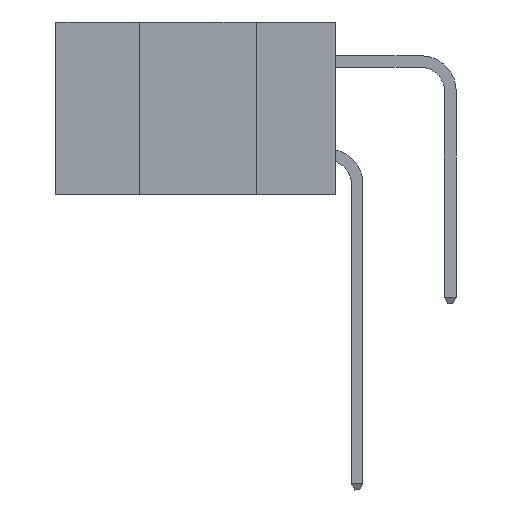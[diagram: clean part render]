
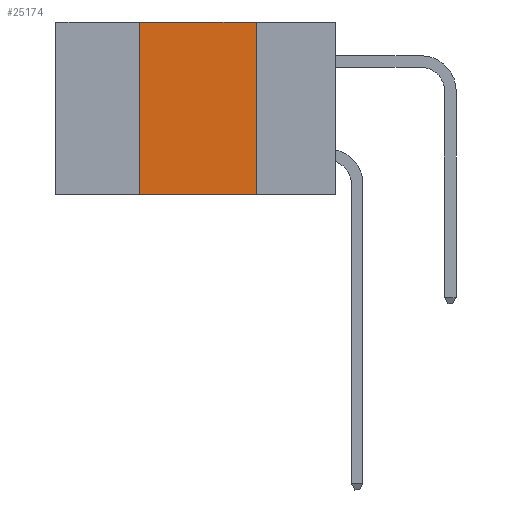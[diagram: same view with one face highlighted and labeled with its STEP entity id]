
A CAD part, left-side view. The second image highlights one B-rep face of the part: STEP entity #25174.
In plain terms, the highlighted planar face has unit normal (-1, 0, 0).
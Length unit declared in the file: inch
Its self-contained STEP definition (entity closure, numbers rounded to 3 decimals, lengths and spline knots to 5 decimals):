
#180 = CARTESIAN_POINT ( 'NONE',  ( 0., 0.42, -0.37 ) ) ;
#3259 = FACE_OUTER_BOUND ( 'NONE', #9190, .T. ) ;
#3650 = AXIS2_PLACEMENT_3D ( 'NONE', #17497, #11956, #22484 ) ;
#5127 = DIRECTION ( 'NONE',  ( 0., 0., -1. ) ) ;
#6590 = CARTESIAN_POINT ( 'NONE',  ( 0., 0.6, 0. ) ) ;
#7867 = LINE ( 'NONE', #29568, #27215 ) ;
#8595 = VERTEX_POINT ( 'NONE', #17747 ) ;
#9190 = EDGE_LOOP ( 'NONE', ( #14017, #14100, #24535, #16120 ) ) ;
#11164 = VECTOR ( 'NONE', #32079, 39.37008 ) ;
#11956 = DIRECTION ( 'NONE',  ( 1., 0., 0. ) ) ;
#12227 = EDGE_CURVE ( 'NONE', #27423, #13908, #7867, .T. ) ;
#12720 = CARTESIAN_POINT ( 'NONE',  ( 0., 0.17, 0. ) ) ;
#13908 = VERTEX_POINT ( 'NONE', #24430 ) ;
#14017 = ORIENTED_EDGE ( 'NONE', *, *, #29795, .F. ) ;
#14100 = ORIENTED_EDGE ( 'NONE', *, *, #14799, .F. ) ;
#14257 = VECTOR ( 'NONE', #5127, 39.37008 ) ;
#14799 = EDGE_CURVE ( 'NONE', #15131, #8595, #25459, .T. ) ;
#14901 = PLANE ( 'NONE',  #3650 ) ;
#15131 = VERTEX_POINT ( 'NONE', #29104 ) ;
#16120 = ORIENTED_EDGE ( 'NONE', *, *, #12227, .T. ) ;
#17497 = CARTESIAN_POINT ( 'NONE',  ( 0., 0.6, 0. ) ) ;
#17747 = CARTESIAN_POINT ( 'NONE',  ( 0., 0.17, 0. ) ) ;
#18653 = EDGE_CURVE ( 'NONE', #27423, #15131, #31736, .T. ) ;
#21730 = CARTESIAN_POINT ( 'NONE',  ( 0., 0.42, 0. ) ) ;
#21853 = DIRECTION ( 'NONE',  ( 0., -1., 0. ) ) ;
#22484 = DIRECTION ( 'NONE',  ( 0., 0., -1. ) ) ;
#22646 = VECTOR ( 'NONE', #21853, 39.37008 ) ;
#24430 = CARTESIAN_POINT ( 'NONE',  ( 0., 0.17, -0.37 ) ) ;
#24535 = ORIENTED_EDGE ( 'NONE', *, *, #18653, .F. ) ;
#25174 = ADVANCED_FACE ( 'NONE', ( #3259 ), #14901, .F. ) ;
#25459 = LINE ( 'NONE', #6590, #22646 ) ;
#27215 = VECTOR ( 'NONE', #29790, 39.37008 ) ;
#27423 = VERTEX_POINT ( 'NONE', #180 ) ;
#28728 = LINE ( 'NONE', #12720, #14257 ) ;
#29104 = CARTESIAN_POINT ( 'NONE',  ( 0., 0.42, 0. ) ) ;
#29568 = CARTESIAN_POINT ( 'NONE',  ( 0., 0.6, -0.37 ) ) ;
#29790 = DIRECTION ( 'NONE',  ( 0., -1., 0. ) ) ;
#29795 = EDGE_CURVE ( 'NONE', #8595, #13908, #28728, .T. ) ;
#31736 = LINE ( 'NONE', #21730, #11164 ) ;
#32079 = DIRECTION ( 'NONE',  ( 0., 0., 1. ) ) ;
